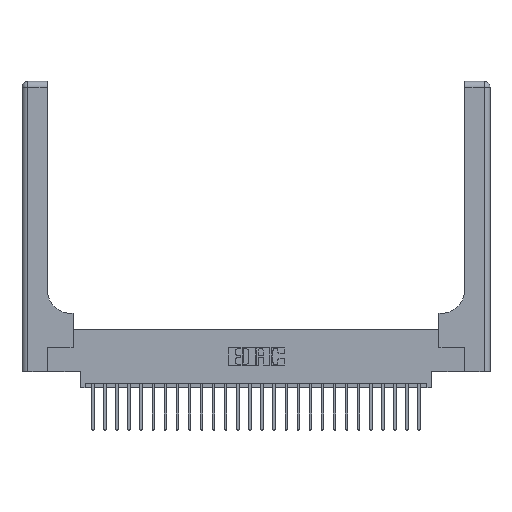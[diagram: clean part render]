
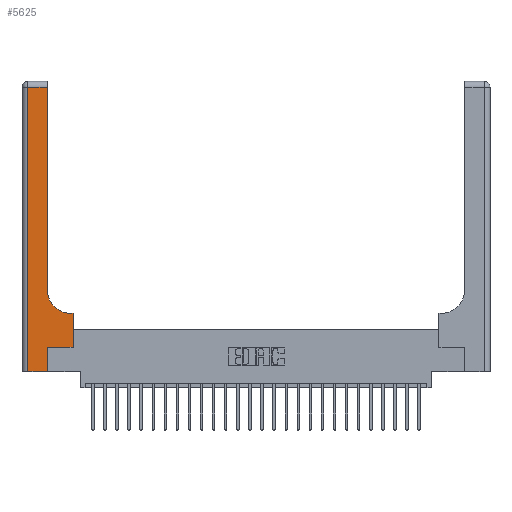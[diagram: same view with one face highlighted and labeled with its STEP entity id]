
A CAD part, top view. The second image highlights one B-rep face of the part: STEP entity #5625.
In plain terms, the highlighted planar face has unit normal (0, 0, 1).
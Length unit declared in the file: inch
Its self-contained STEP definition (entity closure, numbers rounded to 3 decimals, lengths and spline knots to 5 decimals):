
#648 = EDGE_CURVE ( 'NONE', #17451, #22541, #19239, .T. ) ;
#944 = CARTESIAN_POINT ( 'NONE',  ( 0.51, 0.6, 0.37 ) ) ;
#1074 = VERTEX_POINT ( 'NONE', #944 ) ;
#1141 = VECTOR ( 'NONE', #6934, 39.37008 ) ;
#1441 = ORIENTED_EDGE ( 'NONE', *, *, #11035, .T. ) ;
#1660 = CARTESIAN_POINT ( 'NONE',  ( 0.26, 3., 0.37 ) ) ;
#2335 = ORIENTED_EDGE ( 'NONE', *, *, #23131, .T. ) ;
#3099 = LINE ( 'NONE', #10895, #20475 ) ;
#3786 = DIRECTION ( 'NONE',  ( 0., 0., -1. ) ) ;
#4497 = LINE ( 'NONE', #8582, #15626 ) ;
#5019 = CARTESIAN_POINT ( 'NONE',  ( 0.265, 0.25, 0.37 ) ) ;
#5625 = ADVANCED_FACE ( 'NONE', ( #13921 ), #16020, .F. ) ;
#6206 = VECTOR ( 'NONE', #17295, 39.37008 ) ;
#6877 = VERTEX_POINT ( 'NONE', #13268 ) ;
#6934 = DIRECTION ( 'NONE',  ( 1., 0., 0. ) ) ;
#6998 = CARTESIAN_POINT ( 'NONE',  ( 0.06, 0., 0.37 ) ) ;
#7011 = VECTOR ( 'NONE', #11478, 39.37008 ) ;
#7037 = ORIENTED_EDGE ( 'NONE', *, *, #24488, .T. ) ;
#7278 = DIRECTION ( 'NONE',  ( 0., 0., -1. ) ) ;
#7406 = CARTESIAN_POINT ( 'NONE',  ( 0.51, 0.85, 0.37 ) ) ;
#7849 = CARTESIAN_POINT ( 'NONE',  ( 0.26, 2.94, 0.37 ) ) ;
#8582 = CARTESIAN_POINT ( 'NONE',  ( 0.06, 3., 0.37 ) ) ;
#9554 = ORIENTED_EDGE ( 'NONE', *, *, #22102, .T. ) ;
#10087 = CARTESIAN_POINT ( 'NONE',  ( 0.528, 0.25, 0.37 ) ) ;
#10115 = VERTEX_POINT ( 'NONE', #10087 ) ;
#10459 = VERTEX_POINT ( 'NONE', #16874 ) ;
#10895 = CARTESIAN_POINT ( 'NONE',  ( 0.528, 0.25, 0.37 ) ) ;
#10950 = LINE ( 'NONE', #24965, #18739 ) ;
#10956 = VECTOR ( 'NONE', #13208, 39.37008 ) ;
#10960 = CIRCLE ( 'NONE', #18469, 0.25 ) ;
#10980 = CARTESIAN_POINT ( 'NONE',  ( 0., 2.94, 0.37 ) ) ;
#11035 = EDGE_CURVE ( 'NONE', #10459, #1074, #10950, .T. ) ;
#11064 = EDGE_CURVE ( 'NONE', #22541, #10115, #15551, .T. ) ;
#11066 = VERTEX_POINT ( 'NONE', #6998 ) ;
#11281 = CARTESIAN_POINT ( 'NONE',  ( 0., 0., 0.37 ) ) ;
#11478 = DIRECTION ( 'NONE',  ( 1., 0., 0. ) ) ;
#11544 = LINE ( 'NONE', #1660, #17268 ) ;
#11967 = EDGE_CURVE ( 'NONE', #11066, #17451, #25160, .T. ) ;
#12095 = VERTEX_POINT ( 'NONE', #7849 ) ;
#13097 = CARTESIAN_POINT ( 'NONE',  ( 0.265, 0., 0.37 ) ) ;
#13208 = DIRECTION ( 'NONE',  ( -1., 0., 0. ) ) ;
#13268 = CARTESIAN_POINT ( 'NONE',  ( 0.26, 0.85, 0.37 ) ) ;
#13344 = EDGE_CURVE ( 'NONE', #10115, #10459, #3099, .T. ) ;
#13921 = FACE_OUTER_BOUND ( 'NONE', #21029, .T. ) ;
#13937 = CARTESIAN_POINT ( 'NONE',  ( 0.06, 2.94, 0.37 ) ) ;
#15292 = DIRECTION ( 'NONE',  ( -1., 0., 0. ) ) ;
#15551 = LINE ( 'NONE', #5019, #7011 ) ;
#15626 = VECTOR ( 'NONE', #16343, 39.37008 ) ;
#16020 = PLANE ( 'NONE',  #24630 ) ;
#16096 = ORIENTED_EDGE ( 'NONE', *, *, #17253, .T. ) ;
#16226 = DIRECTION ( 'NONE',  ( -1., 0., 0. ) ) ;
#16343 = DIRECTION ( 'NONE',  ( 0., -1., 0. ) ) ;
#16874 = CARTESIAN_POINT ( 'NONE',  ( 0.528, 0.6, 0.37 ) ) ;
#16921 = DIRECTION ( 'NONE',  ( 0., 1., 0. ) ) ;
#17127 = DIRECTION ( 'NONE',  ( 1., 0., 0. ) ) ;
#17253 = EDGE_CURVE ( 'NONE', #12095, #25191, #24866, .T. ) ;
#17268 = VECTOR ( 'NONE', #25429, 39.37008 ) ;
#17295 = DIRECTION ( 'NONE',  ( 0., 1., 0. ) ) ;
#17451 = VERTEX_POINT ( 'NONE', #22222 ) ;
#18087 = ORIENTED_EDGE ( 'NONE', *, *, #648, .T. ) ;
#18469 = AXIS2_PLACEMENT_3D ( 'NONE', #7406, #7278, #17127 ) ;
#18525 = ORIENTED_EDGE ( 'NONE', *, *, #11064, .T. ) ;
#18739 = VECTOR ( 'NONE', #15292, 39.37008 ) ;
#19239 = LINE ( 'NONE', #13097, #6206 ) ;
#19668 = CARTESIAN_POINT ( 'NONE',  ( 0., 3., 0.37 ) ) ;
#20475 = VECTOR ( 'NONE', #16921, 39.37008 ) ;
#21029 = EDGE_LOOP ( 'NONE', ( #7037, #16096, #2335, #25443, #18087, #18525, #22674, #1441, #9554 ) ) ;
#22102 = EDGE_CURVE ( 'NONE', #1074, #6877, #10960, .T. ) ;
#22222 = CARTESIAN_POINT ( 'NONE',  ( 0.265, 0., 0.37 ) ) ;
#22541 = VERTEX_POINT ( 'NONE', #22827 ) ;
#22674 = ORIENTED_EDGE ( 'NONE', *, *, #13344, .T. ) ;
#22827 = CARTESIAN_POINT ( 'NONE',  ( 0.265, 0.25, 0.37 ) ) ;
#23131 = EDGE_CURVE ( 'NONE', #25191, #11066, #4497, .T. ) ;
#24488 = EDGE_CURVE ( 'NONE', #6877, #12095, #11544, .T. ) ;
#24630 = AXIS2_PLACEMENT_3D ( 'NONE', #19668, #3786, #16226 ) ;
#24866 = LINE ( 'NONE', #10980, #10956 ) ;
#24965 = CARTESIAN_POINT ( 'NONE',  ( 0.26, 0.6, 0.37 ) ) ;
#25160 = LINE ( 'NONE', #11281, #1141 ) ;
#25191 = VERTEX_POINT ( 'NONE', #13937 ) ;
#25429 = DIRECTION ( 'NONE',  ( 0., 1., 0. ) ) ;
#25443 = ORIENTED_EDGE ( 'NONE', *, *, #11967, .T. ) ;
